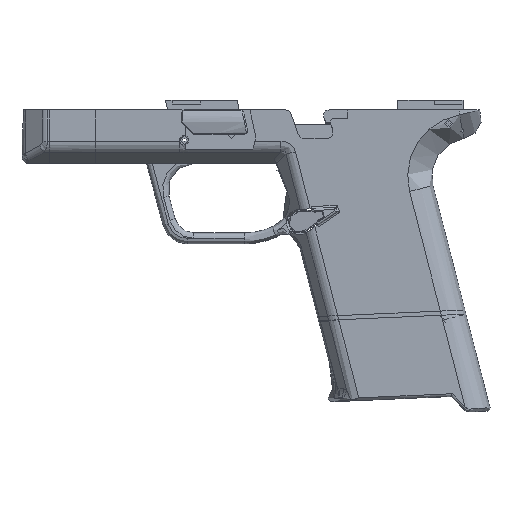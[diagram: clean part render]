
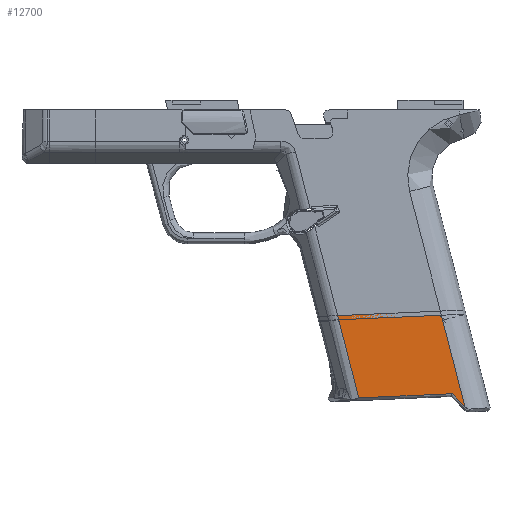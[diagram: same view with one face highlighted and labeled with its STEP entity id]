
A CAD part, left-side view. The second image highlights one B-rep face of the part: STEP entity #12700.
In plain terms, the highlighted face is planar.
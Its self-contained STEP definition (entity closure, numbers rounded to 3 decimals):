
#1008=PLANE('',#13915);
#1677=FACE_OUTER_BOUND('',#2414,.T.);
#2414=EDGE_LOOP('',(#11484,#11485,#11486,#11487,#11488));
#3446=LINE('',#23878,#4561);
#3466=LINE('',#24724,#4581);
#3480=LINE('',#25145,#4595);
#3481=LINE('',#25149,#4596);
#3482=LINE('',#25150,#4597);
#4561=VECTOR('',#16914,10.);
#4581=VECTOR('',#17006,10.);
#4595=VECTOR('',#17078,10.);
#4596=VECTOR('',#17083,10.);
#4597=VECTOR('',#17084,10.);
#6072=VERTEX_POINT('',#23856);
#6074=VERTEX_POINT('',#23876);
#6128=VERTEX_POINT('',#24723);
#6147=VERTEX_POINT('',#24986);
#6155=VERTEX_POINT('',#25148);
#7830=EDGE_CURVE('',#6074,#6072,#3446,.T.);
#7912=EDGE_CURVE('',#6128,#6072,#3466,.T.);
#7957=EDGE_CURVE('',#6147,#6074,#3480,.T.);
#7958=EDGE_CURVE('',#6155,#6147,#3481,.T.);
#7959=EDGE_CURVE('',#6155,#6128,#3482,.T.);
#11484=ORIENTED_EDGE('',*,*,#7830,.F.);
#11485=ORIENTED_EDGE('',*,*,#7957,.F.);
#11486=ORIENTED_EDGE('',*,*,#7958,.F.);
#11487=ORIENTED_EDGE('',*,*,#7959,.T.);
#11488=ORIENTED_EDGE('',*,*,#7912,.T.);
#12700=ADVANCED_FACE('',(#1677),#1008,.T.);
#13915=AXIS2_PLACEMENT_3D('',#25147,#17081,#17082);
#16914=DIRECTION('',(0.,0.999,0.044));
#17006=DIRECTION('',(0.,-0.249,0.969));
#17078=DIRECTION('',(0.,0.697,-0.717));
#17081=DIRECTION('center_axis',(1.,0.,0.));
#17082=DIRECTION('ref_axis',(0.,0.999,0.044));
#17083=DIRECTION('',(0.,-0.249,0.969));
#17084=DIRECTION('',(0.,0.999,0.044));
#23856=CARTESIAN_POINT('',(22.175,-44.727,96.906));
#23876=CARTESIAN_POINT('',(22.175,-78.67,95.402));
#23878=CARTESIAN_POINT('',(22.175,-44.598,96.911));
#24723=CARTESIAN_POINT('',(22.175,-37.062,67.087));
#24724=CARTESIAN_POINT('',(22.175,-37.062,67.087));
#24986=CARTESIAN_POINT('',(22.175,-83.249,100.107));
#25145=CARTESIAN_POINT('',(22.175,-73.025,89.603));
#25147=CARTESIAN_POINT('Origin',(22.175,-74.337,65.435));
#25148=CARTESIAN_POINT('',(22.175,-74.337,65.435));
#25149=CARTESIAN_POINT('',(22.175,-74.337,65.435));
#25150=CARTESIAN_POINT('',(22.175,-40.4,66.939));
